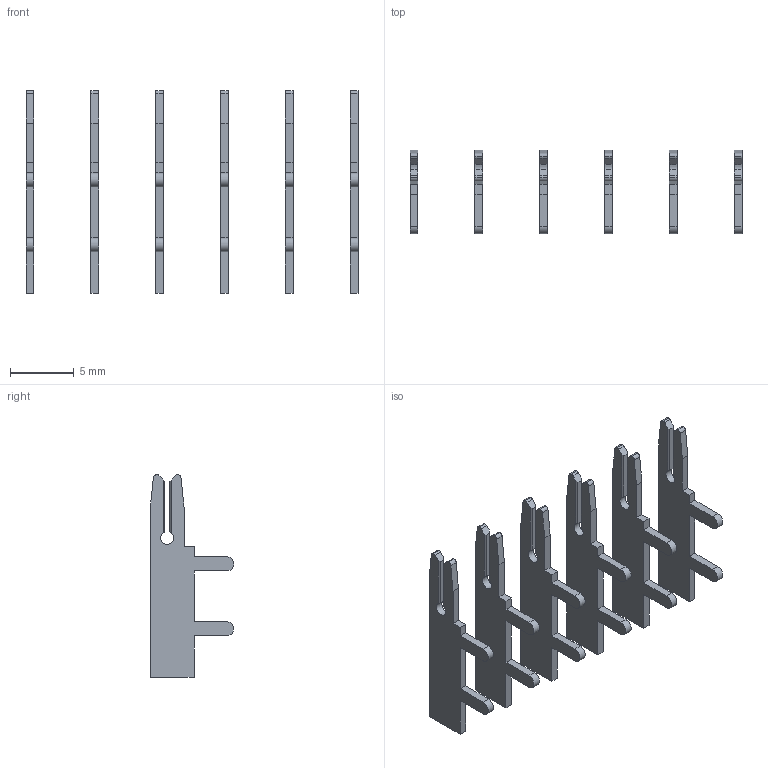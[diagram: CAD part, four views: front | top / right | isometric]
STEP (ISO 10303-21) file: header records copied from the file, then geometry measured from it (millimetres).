
FILE_DESCRIPTION (( 'STEP AP203' ), '1' );
FILE_NAME ('105-006-202-200.STEP', '2020-04-07T22:15:03', ( '' ), ( '' ), 'SwSTEP 2.0', 'SolidWorks 2016', '' );
FILE_SCHEMA (( 'CONFIG_CONTROL_DESIGN' ));
Length unit declared in the file: inch
Products named in the file (2): 100-290-001_100-290-202; 105-006-202-200
Assembly tree (6 placements, depth 2):
  105-006-202-200
    100-290-001_100-290-202  x6
Bounding box: 26 x 6.53 x 15.88 mm (x, y, z)
Volume: 190.6 mm3; surface area: 847.8 mm2
Topology: 6 solids, 6 shells, 180 faces, 504 edges, 336 vertices
Faces by surface type: plane 138, cylinder 42
Entity records: 1322 total; most frequent: CARTESIAN_POINT 191, DIRECTION 172, ORIENTED_EDGE 168, EDGE_CURVE 84, VECTOR 66, LINE 66, VERTEX_POINT 56, AXIS2_PLACEMENT_3D 53
